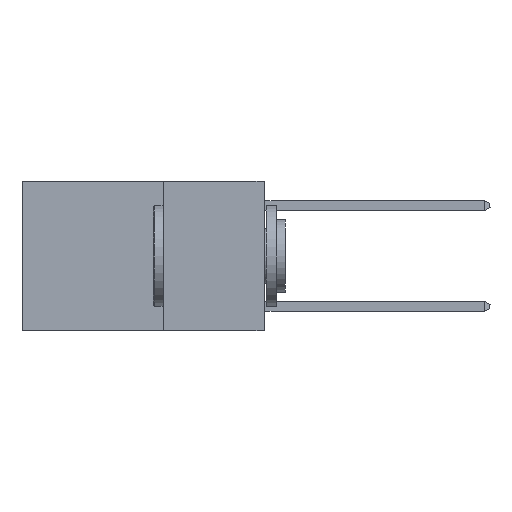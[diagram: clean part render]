
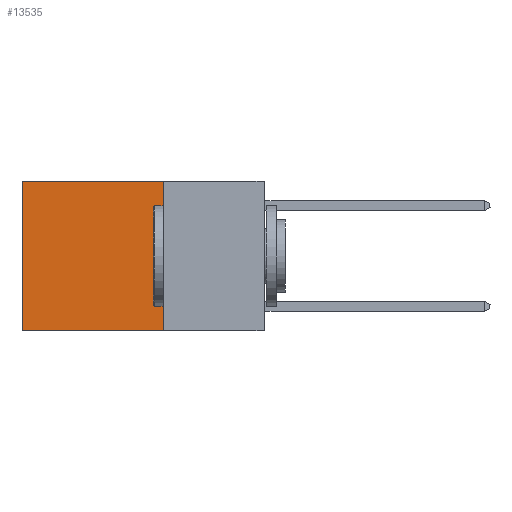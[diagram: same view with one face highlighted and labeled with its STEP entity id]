
A CAD part, left-side view. The second image highlights one B-rep face of the part: STEP entity #13535.
In plain terms, the highlighted planar face has unit normal (-1, 0, 0).
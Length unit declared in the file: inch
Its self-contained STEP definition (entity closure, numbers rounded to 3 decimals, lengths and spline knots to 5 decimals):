
#290 = CARTESIAN_POINT ( 'NONE',  ( 0.2625, 0.6, 0. ) ) ;
#846 = CARTESIAN_POINT ( 'NONE',  ( 0.2625, 0.25, -0.37 ) ) ;
#1281 = PLANE ( 'NONE',  #8042 ) ;
#1557 = ORIENTED_EDGE ( 'NONE', *, *, #19870, .F. ) ;
#2099 = VERTEX_POINT ( 'NONE', #12593 ) ;
#2580 = DIRECTION ( 'NONE',  ( 0., 1., 0. ) ) ;
#3759 = DIRECTION ( 'NONE',  ( 1., 0., 0. ) ) ;
#4453 = EDGE_LOOP ( 'NONE', ( #7396, #1557, #25719, #6348 ) ) ;
#5377 = DIRECTION ( 'NONE',  ( 0., 0., -1. ) ) ;
#5469 = LINE ( 'NONE', #846, #15460 ) ;
#5480 = VERTEX_POINT ( 'NONE', #290 ) ;
#5824 = DIRECTION ( 'NONE',  ( 0., 0., -1. ) ) ;
#6348 = ORIENTED_EDGE ( 'NONE', *, *, #12842, .T. ) ;
#7396 = ORIENTED_EDGE ( 'NONE', *, *, #20857, .T. ) ;
#8042 = AXIS2_PLACEMENT_3D ( 'NONE', #15548, #3759, #20221 ) ;
#8154 = LINE ( 'NONE', #27076, #21860 ) ;
#8252 = FACE_OUTER_BOUND ( 'NONE', #4453, .T. ) ;
#8979 = VECTOR ( 'NONE', #5377, 39.37008 ) ;
#10218 = VERTEX_POINT ( 'NONE', #12565 ) ;
#12163 = CARTESIAN_POINT ( 'NONE',  ( 0.2625, 0.25, 0. ) ) ;
#12552 = EDGE_CURVE ( 'NONE', #10218, #12737, #12972, .T. ) ;
#12565 = CARTESIAN_POINT ( 'NONE',  ( 0.2625, 0.25, 0. ) ) ;
#12593 = CARTESIAN_POINT ( 'NONE',  ( 0.2625, 0.6, -0.37 ) ) ;
#12737 = VERTEX_POINT ( 'NONE', #27866 ) ;
#12842 = EDGE_CURVE ( 'NONE', #10218, #5480, #16834, .T. ) ;
#12972 = LINE ( 'NONE', #26932, #8979 ) ;
#13535 = ADVANCED_FACE ( 'NONE', ( #8252 ), #1281, .F. ) ;
#15460 = VECTOR ( 'NONE', #19751, 39.37008 ) ;
#15548 = CARTESIAN_POINT ( 'NONE',  ( 0.2625, 0.25, 0. ) ) ;
#16834 = LINE ( 'NONE', #12163, #30316 ) ;
#19751 = DIRECTION ( 'NONE',  ( 0., 1., 0. ) ) ;
#19870 = EDGE_CURVE ( 'NONE', #12737, #2099, #5469, .T. ) ;
#20221 = DIRECTION ( 'NONE',  ( 0., 0., -1. ) ) ;
#20857 = EDGE_CURVE ( 'NONE', #5480, #2099, #8154, .T. ) ;
#21860 = VECTOR ( 'NONE', #5824, 39.37008 ) ;
#25719 = ORIENTED_EDGE ( 'NONE', *, *, #12552, .F. ) ;
#26932 = CARTESIAN_POINT ( 'NONE',  ( 0.2625, 0.25, 0. ) ) ;
#27076 = CARTESIAN_POINT ( 'NONE',  ( 0.2625, 0.6, 0. ) ) ;
#27866 = CARTESIAN_POINT ( 'NONE',  ( 0.2625, 0.25, -0.37 ) ) ;
#30316 = VECTOR ( 'NONE', #2580, 39.37008 ) ;
